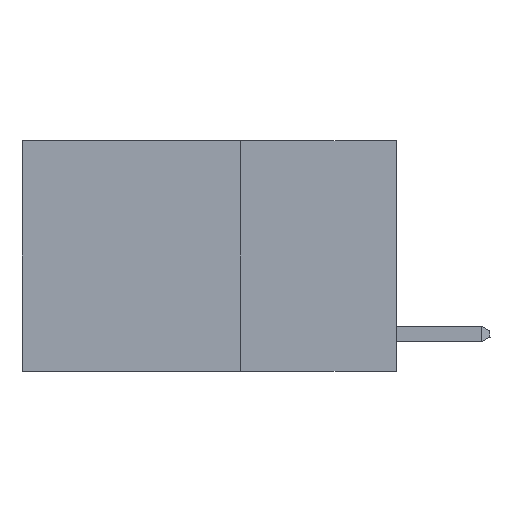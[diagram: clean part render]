
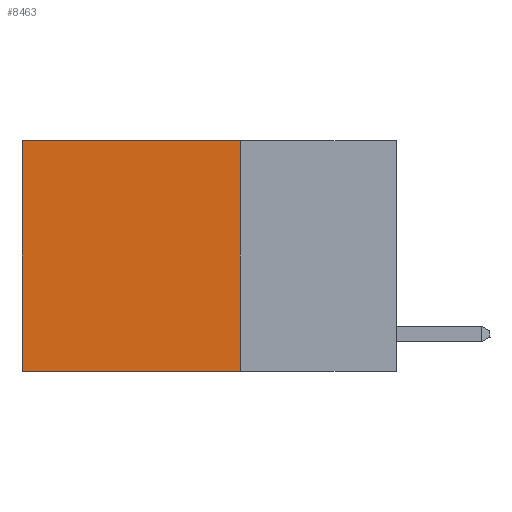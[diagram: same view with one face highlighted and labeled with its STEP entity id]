
A CAD part, left-side view. The second image highlights one B-rep face of the part: STEP entity #8463.
In plain terms, the highlighted planar face has unit normal (-1, 0, 0).
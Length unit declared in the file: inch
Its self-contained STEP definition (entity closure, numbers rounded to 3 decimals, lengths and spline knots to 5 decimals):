
#14 = CARTESIAN_POINT ( 'NONE',  ( 0.2625, 0.25, -0.37 ) ) ;
#253 = CARTESIAN_POINT ( 'NONE',  ( 0.2625, 0.6, -0.37 ) ) ;
#600 = VERTEX_POINT ( 'NONE', #4205 ) ;
#853 = ORIENTED_EDGE ( 'NONE', *, *, #3530, .F. ) ;
#1107 = LINE ( 'NONE', #11127, #10155 ) ;
#1215 = LINE ( 'NONE', #9683, #4028 ) ;
#1220 = DIRECTION ( 'NONE',  ( 0., 1., 0. ) ) ;
#1262 = VERTEX_POINT ( 'NONE', #7872 ) ;
#1268 = VECTOR ( 'NONE', #1220, 39.37008 ) ;
#1578 = FACE_OUTER_BOUND ( 'NONE', #8623, .T. ) ;
#1630 = LINE ( 'NONE', #14, #1268 ) ;
#2832 = DIRECTION ( 'NONE',  ( 1., 0., 0. ) ) ;
#3020 = CARTESIAN_POINT ( 'NONE',  ( 0.2625, 0.25, 0. ) ) ;
#3530 = EDGE_CURVE ( 'NONE', #1262, #600, #1215, .T. ) ;
#4028 = VECTOR ( 'NONE', #12948, 39.37008 ) ;
#4205 = CARTESIAN_POINT ( 'NONE',  ( 0.2625, 0.25, -0.37 ) ) ;
#4629 = VERTEX_POINT ( 'NONE', #14801 ) ;
#4699 = AXIS2_PLACEMENT_3D ( 'NONE', #8809, #2832, #11032 ) ;
#5815 = EDGE_CURVE ( 'NONE', #1262, #4629, #9657, .T. ) ;
#6113 = ORIENTED_EDGE ( 'NONE', *, *, #6692, .T. ) ;
#6692 = EDGE_CURVE ( 'NONE', #4629, #11264, #1107, .T. ) ;
#7114 = EDGE_CURVE ( 'NONE', #600, #11264, #1630, .T. ) ;
#7872 = CARTESIAN_POINT ( 'NONE',  ( 0.2625, 0.25, 0. ) ) ;
#8463 = ADVANCED_FACE ( 'NONE', ( #1578 ), #14277, .F. ) ;
#8623 = EDGE_LOOP ( 'NONE', ( #6113, #12174, #853, #10278 ) ) ;
#8809 = CARTESIAN_POINT ( 'NONE',  ( 0.2625, 0.25, 0. ) ) ;
#9317 = VECTOR ( 'NONE', #13364, 39.37008 ) ;
#9657 = LINE ( 'NONE', #3020, #9317 ) ;
#9683 = CARTESIAN_POINT ( 'NONE',  ( 0.2625, 0.25, 0. ) ) ;
#10155 = VECTOR ( 'NONE', #12234, 39.37008 ) ;
#10278 = ORIENTED_EDGE ( 'NONE', *, *, #5815, .T. ) ;
#11032 = DIRECTION ( 'NONE',  ( 0., 0., -1. ) ) ;
#11127 = CARTESIAN_POINT ( 'NONE',  ( 0.2625, 0.6, 0. ) ) ;
#11264 = VERTEX_POINT ( 'NONE', #253 ) ;
#12174 = ORIENTED_EDGE ( 'NONE', *, *, #7114, .F. ) ;
#12234 = DIRECTION ( 'NONE',  ( 0., 0., -1. ) ) ;
#12948 = DIRECTION ( 'NONE',  ( 0., 0., -1. ) ) ;
#13364 = DIRECTION ( 'NONE',  ( 0., 1., 0. ) ) ;
#14277 = PLANE ( 'NONE',  #4699 ) ;
#14801 = CARTESIAN_POINT ( 'NONE',  ( 0.2625, 0.6, 0. ) ) ;
